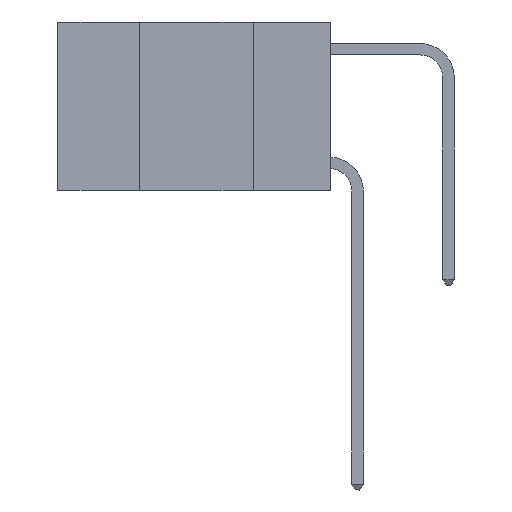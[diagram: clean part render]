
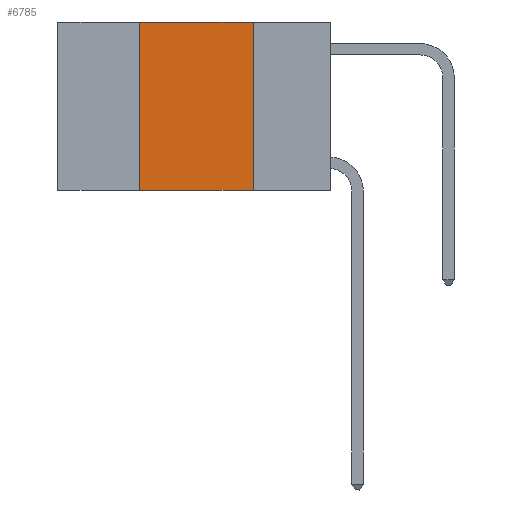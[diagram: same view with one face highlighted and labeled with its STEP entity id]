
A CAD part, left-side view. The second image highlights one B-rep face of the part: STEP entity #6785.
In plain terms, the highlighted planar face has unit normal (-1, 0, 0).
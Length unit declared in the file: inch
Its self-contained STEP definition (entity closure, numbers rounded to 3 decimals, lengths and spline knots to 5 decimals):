
#89 = EDGE_LOOP ( 'NONE', ( #4827, #13035, #4193, #26087 ) ) ;
#748 = DIRECTION ( 'NONE',  ( 1., 0., 0. ) ) ;
#1037 = DIRECTION ( 'NONE',  ( 0., 0., -1. ) ) ;
#2921 = DIRECTION ( 'NONE',  ( 0., 0., -1. ) ) ;
#4193 = ORIENTED_EDGE ( 'NONE', *, *, #13312, .F. ) ;
#4400 = CARTESIAN_POINT ( 'NONE',  ( 0., 0.6, 0. ) ) ;
#4740 = CARTESIAN_POINT ( 'NONE',  ( 0., 0.17, 0. ) ) ;
#4827 = ORIENTED_EDGE ( 'NONE', *, *, #8280, .F. ) ;
#5242 = AXIS2_PLACEMENT_3D ( 'NONE', #14232, #748, #1037 ) ;
#5415 = LINE ( 'NONE', #14179, #14415 ) ;
#6168 = LINE ( 'NONE', #22175, #20939 ) ;
#6785 = ADVANCED_FACE ( 'NONE', ( #7398 ), #16455, .F. ) ;
#7398 = FACE_OUTER_BOUND ( 'NONE', #89, .T. ) ;
#8280 = EDGE_CURVE ( 'NONE', #26598, #19975, #5415, .T. ) ;
#11690 = VERTEX_POINT ( 'NONE', #22891 ) ;
#12313 = DIRECTION ( 'NONE',  ( 0., 0., 1. ) ) ;
#12459 = CARTESIAN_POINT ( 'NONE',  ( 0., 0.42, 0. ) ) ;
#13035 = ORIENTED_EDGE ( 'NONE', *, *, #17858, .F. ) ;
#13312 = EDGE_CURVE ( 'NONE', #29178, #11690, #23587, .T. ) ;
#14179 = CARTESIAN_POINT ( 'NONE',  ( 0., 0.17, 0. ) ) ;
#14232 = CARTESIAN_POINT ( 'NONE',  ( 0., 0.6, 0. ) ) ;
#14415 = VECTOR ( 'NONE', #2921, 39.37008 ) ;
#14765 = DIRECTION ( 'NONE',  ( 0., -1., 0. ) ) ;
#15678 = DIRECTION ( 'NONE',  ( 0., -1., 0. ) ) ;
#16455 = PLANE ( 'NONE',  #5242 ) ;
#17858 = EDGE_CURVE ( 'NONE', #11690, #26598, #22340, .T. ) ;
#19975 = VERTEX_POINT ( 'NONE', #23183 ) ;
#20939 = VECTOR ( 'NONE', #14765, 39.37008 ) ;
#20998 = EDGE_CURVE ( 'NONE', #29178, #19975, #6168, .T. ) ;
#22175 = CARTESIAN_POINT ( 'NONE',  ( 0., 0.6, -0.37 ) ) ;
#22340 = LINE ( 'NONE', #4400, #23737 ) ;
#22891 = CARTESIAN_POINT ( 'NONE',  ( 0., 0.42, 0. ) ) ;
#23183 = CARTESIAN_POINT ( 'NONE',  ( 0., 0.17, -0.37 ) ) ;
#23587 = LINE ( 'NONE', #12459, #28761 ) ;
#23737 = VECTOR ( 'NONE', #15678, 39.37008 ) ;
#24079 = CARTESIAN_POINT ( 'NONE',  ( 0., 0.42, -0.37 ) ) ;
#26087 = ORIENTED_EDGE ( 'NONE', *, *, #20998, .T. ) ;
#26598 = VERTEX_POINT ( 'NONE', #4740 ) ;
#28761 = VECTOR ( 'NONE', #12313, 39.37008 ) ;
#29178 = VERTEX_POINT ( 'NONE', #24079 ) ;
